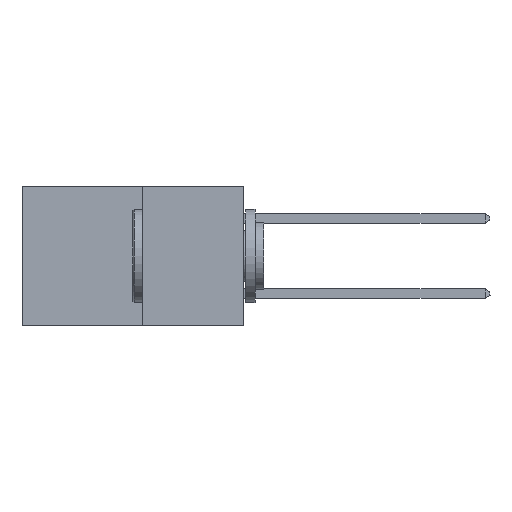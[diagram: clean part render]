
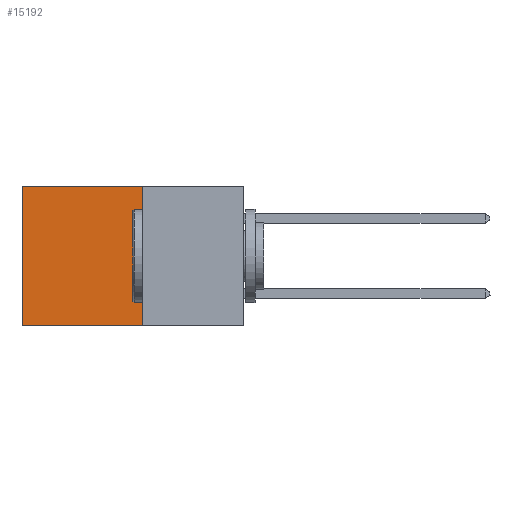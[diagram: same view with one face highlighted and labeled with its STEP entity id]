
A CAD part, left-side view. The second image highlights one B-rep face of the part: STEP entity #15192.
In plain terms, the highlighted planar face has unit normal (-1, 0, 0).
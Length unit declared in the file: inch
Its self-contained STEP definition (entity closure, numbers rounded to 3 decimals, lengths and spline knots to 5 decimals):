
#593 = DIRECTION ( 'NONE',  ( 0., 0., -1. ) ) ;
#734 = PLANE ( 'NONE',  #1976 ) ;
#963 = EDGE_CURVE ( 'NONE', #20516, #21621, #4390, .T. ) ;
#1976 = AXIS2_PLACEMENT_3D ( 'NONE', #11466, #13273, #2549 ) ;
#2220 = VECTOR ( 'NONE', #4290, 39.37008 ) ;
#2267 = VECTOR ( 'NONE', #14131, 39.37008 ) ;
#2549 = DIRECTION ( 'NONE',  ( 0., 0., -1. ) ) ;
#2788 = LINE ( 'NONE', #11376, #2220 ) ;
#3180 = VERTEX_POINT ( 'NONE', #11885 ) ;
#4290 = DIRECTION ( 'NONE',  ( 0., 1., 0. ) ) ;
#4390 = LINE ( 'NONE', #7830, #9161 ) ;
#4745 = LINE ( 'NONE', #13416, #19921 ) ;
#4866 = ORIENTED_EDGE ( 'NONE', *, *, #12410, .T. ) ;
#6460 = CARTESIAN_POINT ( 'NONE',  ( 0.277, 0.59, -0.37 ) ) ;
#7072 = LINE ( 'NONE', #22839, #2267 ) ;
#7830 = CARTESIAN_POINT ( 'NONE',  ( 0.277, 0.27, -0.37 ) ) ;
#8625 = EDGE_LOOP ( 'NONE', ( #18972, #10588, #10751, #4866 ) ) ;
#9161 = VECTOR ( 'NONE', #593, 39.37008 ) ;
#10588 = ORIENTED_EDGE ( 'NONE', *, *, #12509, .F. ) ;
#10751 = ORIENTED_EDGE ( 'NONE', *, *, #963, .F. ) ;
#11347 = FACE_OUTER_BOUND ( 'NONE', #8625, .T. ) ;
#11376 = CARTESIAN_POINT ( 'NONE',  ( 0.277, 0.27, 0. ) ) ;
#11466 = CARTESIAN_POINT ( 'NONE',  ( 0.277, 0.27, -0.37 ) ) ;
#11493 = EDGE_CURVE ( 'NONE', #3180, #13262, #7072, .T. ) ;
#11885 = CARTESIAN_POINT ( 'NONE',  ( 0.277, 0.59, 0. ) ) ;
#12410 = EDGE_CURVE ( 'NONE', #20516, #3180, #2788, .T. ) ;
#12509 = EDGE_CURVE ( 'NONE', #21621, #13262, #4745, .T. ) ;
#13262 = VERTEX_POINT ( 'NONE', #6460 ) ;
#13273 = DIRECTION ( 'NONE',  ( 1., 0., 0. ) ) ;
#13416 = CARTESIAN_POINT ( 'NONE',  ( 0.277, 0.27, -0.37 ) ) ;
#14131 = DIRECTION ( 'NONE',  ( 0., 0., -1. ) ) ;
#15192 = ADVANCED_FACE ( 'NONE', ( #11347 ), #734, .F. ) ;
#16861 = DIRECTION ( 'NONE',  ( 0., 1., 0. ) ) ;
#18580 = CARTESIAN_POINT ( 'NONE',  ( 0.277, 0.27, -0.37 ) ) ;
#18972 = ORIENTED_EDGE ( 'NONE', *, *, #11493, .T. ) ;
#19921 = VECTOR ( 'NONE', #16861, 39.37008 ) ;
#20516 = VERTEX_POINT ( 'NONE', #20833 ) ;
#20833 = CARTESIAN_POINT ( 'NONE',  ( 0.277, 0.27, 0. ) ) ;
#21621 = VERTEX_POINT ( 'NONE', #18580 ) ;
#22839 = CARTESIAN_POINT ( 'NONE',  ( 0.277, 0.59, -0.37 ) ) ;
